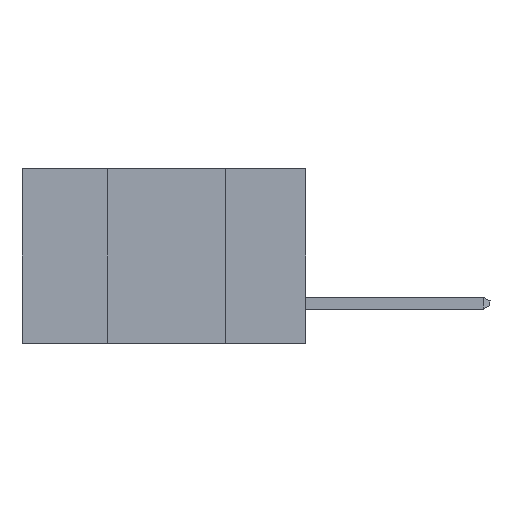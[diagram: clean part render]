
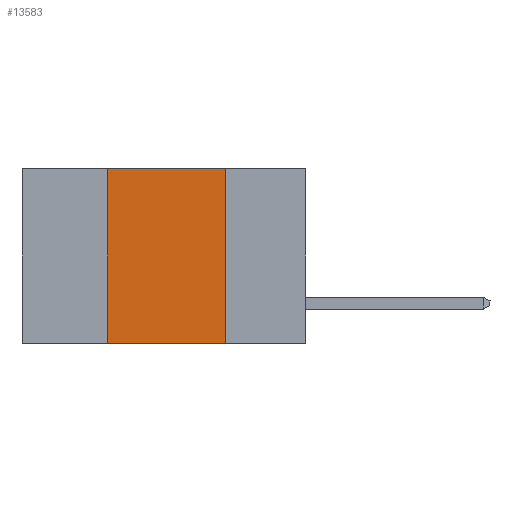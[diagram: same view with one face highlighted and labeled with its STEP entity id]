
A CAD part, left-side view. The second image highlights one B-rep face of the part: STEP entity #13583.
In plain terms, the highlighted planar face has unit normal (-1, 0, 0).
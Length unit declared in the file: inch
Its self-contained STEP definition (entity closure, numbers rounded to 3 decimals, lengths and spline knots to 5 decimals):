
#1164 = VERTEX_POINT ( 'NONE', #19007 ) ;
#2141 = EDGE_CURVE ( 'NONE', #6181, #4429, #5519, .T. ) ;
#2761 = ORIENTED_EDGE ( 'NONE', *, *, #12891, .F. ) ;
#3092 = PLANE ( 'NONE',  #8367 ) ;
#3606 = ORIENTED_EDGE ( 'NONE', *, *, #6571, .F. ) ;
#4215 = ORIENTED_EDGE ( 'NONE', *, *, #9099, .F. ) ;
#4429 = VERTEX_POINT ( 'NONE', #14806 ) ;
#4803 = DIRECTION ( 'NONE',  ( 0., 0., -1. ) ) ;
#5081 = LINE ( 'NONE', #6562, #21798 ) ;
#5519 = LINE ( 'NONE', #5863, #8510 ) ;
#5749 = DIRECTION ( 'NONE',  ( 0., -1., 0. ) ) ;
#5863 = CARTESIAN_POINT ( 'NONE',  ( 0., 0.6, -0.37 ) ) ;
#6042 = DIRECTION ( 'NONE',  ( 0., 0., 1. ) ) ;
#6170 = CARTESIAN_POINT ( 'NONE',  ( 0., 0.42, -0.37 ) ) ;
#6181 = VERTEX_POINT ( 'NONE', #6170 ) ;
#6562 = CARTESIAN_POINT ( 'NONE',  ( 0., 0.17, -0.37 ) ) ;
#6571 = EDGE_CURVE ( 'NONE', #1164, #15728, #10731, .T. ) ;
#7232 = EDGE_LOOP ( 'NONE', ( #2761, #3606, #4215, #8451 ) ) ;
#8122 = CARTESIAN_POINT ( 'NONE',  ( 0., 0.6, 0. ) ) ;
#8147 = VECTOR ( 'NONE', #15850, 39.37008 ) ;
#8367 = AXIS2_PLACEMENT_3D ( 'NONE', #8122, #18806, #4803 ) ;
#8451 = ORIENTED_EDGE ( 'NONE', *, *, #2141, .T. ) ;
#8510 = VECTOR ( 'NONE', #5749, 39.37008 ) ;
#8888 = CARTESIAN_POINT ( 'NONE',  ( 0., 0.6, 0. ) ) ;
#9099 = EDGE_CURVE ( 'NONE', #6181, #1164, #13315, .T. ) ;
#10731 = LINE ( 'NONE', #8888, #8147 ) ;
#11532 = FACE_OUTER_BOUND ( 'NONE', #7232, .T. ) ;
#12025 = DIRECTION ( 'NONE',  ( 0., 0., -1. ) ) ;
#12891 = EDGE_CURVE ( 'NONE', #15728, #4429, #5081, .T. ) ;
#13315 = LINE ( 'NONE', #14813, #19832 ) ;
#13583 = ADVANCED_FACE ( 'NONE', ( #11532 ), #3092, .F. ) ;
#14806 = CARTESIAN_POINT ( 'NONE',  ( 0., 0.17, -0.37 ) ) ;
#14813 = CARTESIAN_POINT ( 'NONE',  ( 0., 0.42, -0.37 ) ) ;
#15362 = CARTESIAN_POINT ( 'NONE',  ( 0., 0.17, 0. ) ) ;
#15728 = VERTEX_POINT ( 'NONE', #15362 ) ;
#15850 = DIRECTION ( 'NONE',  ( 0., -1., 0. ) ) ;
#18806 = DIRECTION ( 'NONE',  ( 1., 0., 0. ) ) ;
#19007 = CARTESIAN_POINT ( 'NONE',  ( 0., 0.42, 0. ) ) ;
#19832 = VECTOR ( 'NONE', #6042, 39.37008 ) ;
#21798 = VECTOR ( 'NONE', #12025, 39.37008 ) ;
